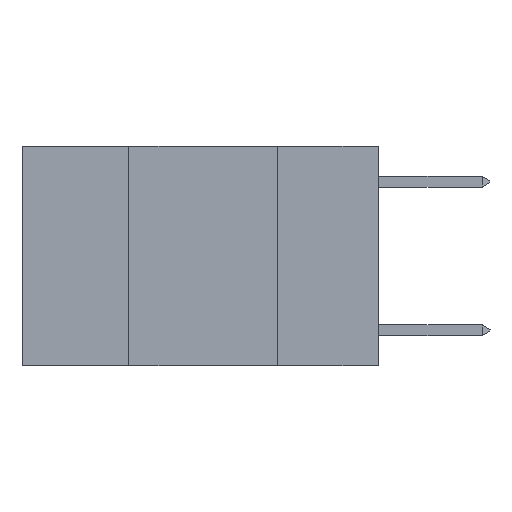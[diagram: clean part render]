
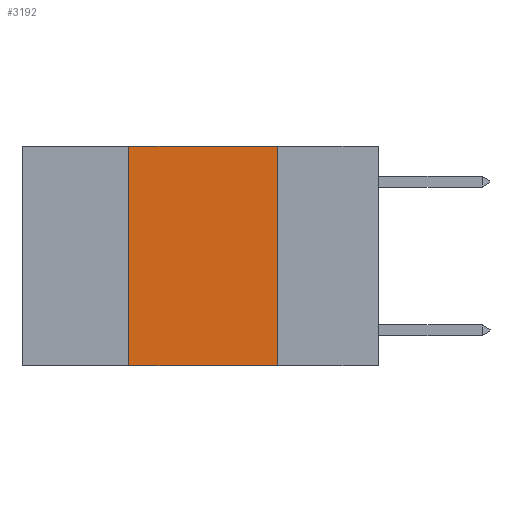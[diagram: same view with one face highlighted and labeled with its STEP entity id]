
A CAD part, left-side view. The second image highlights one B-rep face of the part: STEP entity #3192.
In plain terms, the highlighted planar face has unit normal (-1, 0, 0).
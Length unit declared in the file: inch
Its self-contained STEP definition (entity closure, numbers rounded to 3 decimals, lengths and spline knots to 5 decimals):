
#378 = EDGE_LOOP ( 'NONE', ( #979, #12500, #2360, #6970 ) ) ;
#458 = EDGE_CURVE ( 'NONE', #1837, #10303, #2254, .T. ) ;
#979 = ORIENTED_EDGE ( 'NONE', *, *, #458, .F. ) ;
#1052 = CARTESIAN_POINT ( 'NONE',  ( 0., 0.42, 0. ) ) ;
#1134 = DIRECTION ( 'NONE',  ( 0., -1., 0. ) ) ;
#1171 = CARTESIAN_POINT ( 'NONE',  ( 0., 0.42, -0.37 ) ) ;
#1837 = VERTEX_POINT ( 'NONE', #2252 ) ;
#1891 = DIRECTION ( 'NONE',  ( 0., 0., -1. ) ) ;
#1952 = DIRECTION ( 'NONE',  ( 0., -1., 0. ) ) ;
#1995 = VECTOR ( 'NONE', #8738, 39.37008 ) ;
#2252 = CARTESIAN_POINT ( 'NONE',  ( 0., 0.17, 0. ) ) ;
#2254 = LINE ( 'NONE', #10907, #4632 ) ;
#2306 = CARTESIAN_POINT ( 'NONE',  ( 0., 0.17, -0.37 ) ) ;
#2360 = ORIENTED_EDGE ( 'NONE', *, *, #7323, .F. ) ;
#2682 = VERTEX_POINT ( 'NONE', #1171 ) ;
#3192 = ADVANCED_FACE ( 'NONE', ( #6940 ), #12756, .F. ) ;
#3254 = AXIS2_PLACEMENT_3D ( 'NONE', #5880, #7868, #1891 ) ;
#3967 = CARTESIAN_POINT ( 'NONE',  ( 0., 0.6, -0.37 ) ) ;
#4632 = VECTOR ( 'NONE', #9734, 39.37008 ) ;
#5296 = EDGE_CURVE ( 'NONE', #8206, #1837, #10172, .T. ) ;
#5794 = VECTOR ( 'NONE', #1952, 39.37008 ) ;
#5880 = CARTESIAN_POINT ( 'NONE',  ( 0., 0.6, 0. ) ) ;
#6144 = EDGE_CURVE ( 'NONE', #2682, #10303, #8443, .T. ) ;
#6940 = FACE_OUTER_BOUND ( 'NONE', #378, .T. ) ;
#6970 = ORIENTED_EDGE ( 'NONE', *, *, #6144, .T. ) ;
#7163 = CARTESIAN_POINT ( 'NONE',  ( 0., 0.6, 0. ) ) ;
#7323 = EDGE_CURVE ( 'NONE', #2682, #8206, #9948, .T. ) ;
#7508 = VECTOR ( 'NONE', #1134, 39.37008 ) ;
#7868 = DIRECTION ( 'NONE',  ( 1., 0., 0. ) ) ;
#8206 = VERTEX_POINT ( 'NONE', #1052 ) ;
#8443 = LINE ( 'NONE', #3967, #5794 ) ;
#8738 = DIRECTION ( 'NONE',  ( 0., 0., 1. ) ) ;
#9734 = DIRECTION ( 'NONE',  ( 0., 0., -1. ) ) ;
#9948 = LINE ( 'NONE', #12698, #1995 ) ;
#10172 = LINE ( 'NONE', #7163, #7508 ) ;
#10303 = VERTEX_POINT ( 'NONE', #2306 ) ;
#10907 = CARTESIAN_POINT ( 'NONE',  ( 0., 0.17, 0. ) ) ;
#12500 = ORIENTED_EDGE ( 'NONE', *, *, #5296, .F. ) ;
#12698 = CARTESIAN_POINT ( 'NONE',  ( 0., 0.42, 0. ) ) ;
#12756 = PLANE ( 'NONE',  #3254 ) ;
